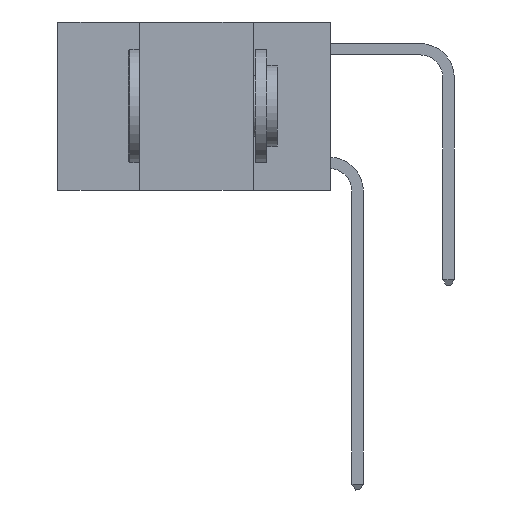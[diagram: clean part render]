
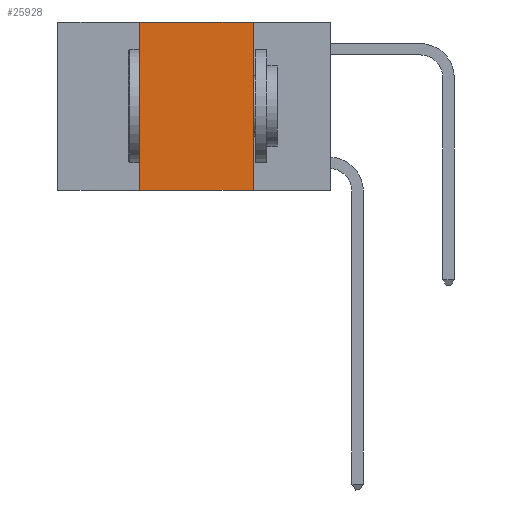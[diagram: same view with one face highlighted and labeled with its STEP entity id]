
A CAD part, left-side view. The second image highlights one B-rep face of the part: STEP entity #25928.
In plain terms, the highlighted planar face has unit normal (-1, 0, 0).
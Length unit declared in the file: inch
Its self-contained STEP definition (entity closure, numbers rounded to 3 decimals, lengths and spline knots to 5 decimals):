
#1983 = LINE ( 'NONE', #32256, #7705 ) ;
#2108 = CARTESIAN_POINT ( 'NONE',  ( 0., 0.42, 0. ) ) ;
#2156 = LINE ( 'NONE', #17050, #26052 ) ;
#3292 = VECTOR ( 'NONE', #26031, 39.37008 ) ;
#4100 = DIRECTION ( 'NONE',  ( 0., 0., -1. ) ) ;
#4346 = DIRECTION ( 'NONE',  ( 0., 0., -1. ) ) ;
#5622 = ORIENTED_EDGE ( 'NONE', *, *, #30533, .F. ) ;
#5924 = LINE ( 'NONE', #19004, #31544 ) ;
#7705 = VECTOR ( 'NONE', #12211, 39.37008 ) ;
#8672 = EDGE_CURVE ( 'NONE', #15156, #14892, #5924, .T. ) ;
#9875 = VERTEX_POINT ( 'NONE', #17861 ) ;
#10575 = VERTEX_POINT ( 'NONE', #29973 ) ;
#11131 = PLANE ( 'NONE',  #14944 ) ;
#12211 = DIRECTION ( 'NONE',  ( 0., -1., 0. ) ) ;
#13342 = ORIENTED_EDGE ( 'NONE', *, *, #20529, .F. ) ;
#14425 = EDGE_CURVE ( 'NONE', #15156, #9875, #1983, .T. ) ;
#14892 = VERTEX_POINT ( 'NONE', #2108 ) ;
#14944 = AXIS2_PLACEMENT_3D ( 'NONE', #21859, #19354, #4100 ) ;
#15156 = VERTEX_POINT ( 'NONE', #26675 ) ;
#15511 = ORIENTED_EDGE ( 'NONE', *, *, #14425, .T. ) ;
#16155 = FACE_OUTER_BOUND ( 'NONE', #23389, .T. ) ;
#17050 = CARTESIAN_POINT ( 'NONE',  ( 0., 0.17, 0. ) ) ;
#17861 = CARTESIAN_POINT ( 'NONE',  ( 0., 0.17, -0.37 ) ) ;
#19004 = CARTESIAN_POINT ( 'NONE',  ( 0., 0.42, 0. ) ) ;
#19354 = DIRECTION ( 'NONE',  ( 1., 0., 0. ) ) ;
#20529 = EDGE_CURVE ( 'NONE', #10575, #9875, #2156, .T. ) ;
#21859 = CARTESIAN_POINT ( 'NONE',  ( 0., 0.6, 0. ) ) ;
#23389 = EDGE_LOOP ( 'NONE', ( #13342, #5622, #24249, #15511 ) ) ;
#24191 = CARTESIAN_POINT ( 'NONE',  ( 0., 0.6, 0. ) ) ;
#24249 = ORIENTED_EDGE ( 'NONE', *, *, #8672, .F. ) ;
#25928 = ADVANCED_FACE ( 'NONE', ( #16155 ), #11131, .F. ) ;
#26031 = DIRECTION ( 'NONE',  ( 0., -1., 0. ) ) ;
#26052 = VECTOR ( 'NONE', #4346, 39.37008 ) ;
#26675 = CARTESIAN_POINT ( 'NONE',  ( 0., 0.42, -0.37 ) ) ;
#29973 = CARTESIAN_POINT ( 'NONE',  ( 0., 0.17, 0. ) ) ;
#30533 = EDGE_CURVE ( 'NONE', #14892, #10575, #31354, .T. ) ;
#31354 = LINE ( 'NONE', #24191, #3292 ) ;
#31544 = VECTOR ( 'NONE', #31840, 39.37008 ) ;
#31840 = DIRECTION ( 'NONE',  ( 0., 0., 1. ) ) ;
#32256 = CARTESIAN_POINT ( 'NONE',  ( 0., 0.6, -0.37 ) ) ;
